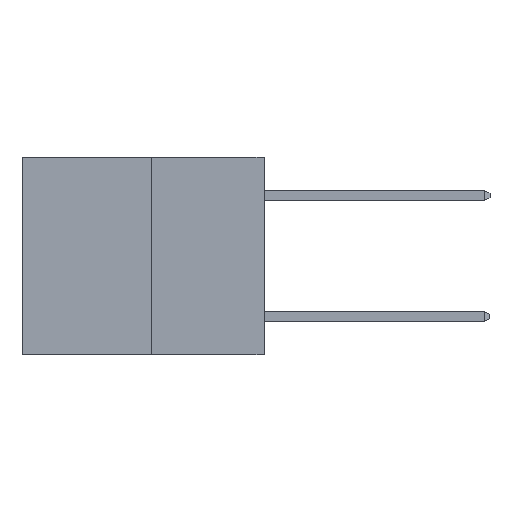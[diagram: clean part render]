
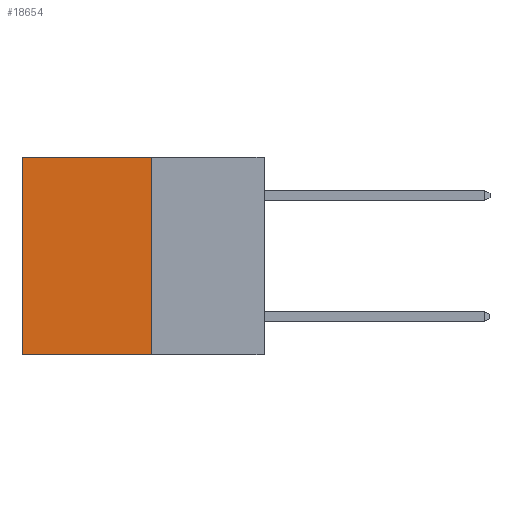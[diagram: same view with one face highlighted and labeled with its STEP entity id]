
A CAD part, left-side view. The second image highlights one B-rep face of the part: STEP entity #18654.
In plain terms, the highlighted planar face has unit normal (-1, 0, 0).
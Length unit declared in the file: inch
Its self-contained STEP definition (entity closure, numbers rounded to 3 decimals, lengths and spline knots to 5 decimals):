
#894 = CARTESIAN_POINT ( 'NONE',  ( 0.3165, 0.6, 0. ) ) ;
#2401 = DIRECTION ( 'NONE',  ( 0., 0., -1. ) ) ;
#2449 = VERTEX_POINT ( 'NONE', #3518 ) ;
#2598 = VECTOR ( 'NONE', #17071, 39.37008 ) ;
#3518 = CARTESIAN_POINT ( 'NONE',  ( 0.3165, 0.28, -0.49 ) ) ;
#3883 = LINE ( 'NONE', #11836, #6253 ) ;
#4028 = EDGE_LOOP ( 'NONE', ( #17519, #9952, #17706, #15901 ) ) ;
#4644 = CARTESIAN_POINT ( 'NONE',  ( 0.3165, 0.28, 0. ) ) ;
#5313 = CARTESIAN_POINT ( 'NONE',  ( 0.3165, 0.6, -0.49 ) ) ;
#6253 = VECTOR ( 'NONE', #16473, 39.37008 ) ;
#6713 = DIRECTION ( 'NONE',  ( 0., 0., -1. ) ) ;
#6855 = EDGE_CURVE ( 'NONE', #7394, #12419, #11944, .T. ) ;
#7394 = VERTEX_POINT ( 'NONE', #17619 ) ;
#7430 = LINE ( 'NONE', #15660, #16113 ) ;
#8497 = PLANE ( 'NONE',  #19822 ) ;
#9324 = EDGE_CURVE ( 'NONE', #7394, #2449, #10800, .T. ) ;
#9455 = FACE_OUTER_BOUND ( 'NONE', #4028, .T. ) ;
#9952 = ORIENTED_EDGE ( 'NONE', *, *, #15131, .F. ) ;
#10045 = CARTESIAN_POINT ( 'NONE',  ( 0.3165, 0.28, -0.49 ) ) ;
#10800 = LINE ( 'NONE', #16528, #17772 ) ;
#11588 = DIRECTION ( 'NONE',  ( 1., 0., 0. ) ) ;
#11836 = CARTESIAN_POINT ( 'NONE',  ( 0.3165, 0.28, -0.49 ) ) ;
#11944 = LINE ( 'NONE', #4644, #2598 ) ;
#12419 = VERTEX_POINT ( 'NONE', #894 ) ;
#15131 = EDGE_CURVE ( 'NONE', #2449, #15538, #3883, .T. ) ;
#15538 = VERTEX_POINT ( 'NONE', #5313 ) ;
#15660 = CARTESIAN_POINT ( 'NONE',  ( 0.3165, 0.6, -0.49 ) ) ;
#15847 = EDGE_CURVE ( 'NONE', #12419, #15538, #7430, .T. ) ;
#15901 = ORIENTED_EDGE ( 'NONE', *, *, #6855, .T. ) ;
#16113 = VECTOR ( 'NONE', #6713, 39.37008 ) ;
#16473 = DIRECTION ( 'NONE',  ( 0., 1., 0. ) ) ;
#16528 = CARTESIAN_POINT ( 'NONE',  ( 0.3165, 0.28, -0.49 ) ) ;
#16669 = DIRECTION ( 'NONE',  ( 0., 0., -1. ) ) ;
#17071 = DIRECTION ( 'NONE',  ( 0., 1., 0. ) ) ;
#17519 = ORIENTED_EDGE ( 'NONE', *, *, #15847, .T. ) ;
#17619 = CARTESIAN_POINT ( 'NONE',  ( 0.3165, 0.28, 0. ) ) ;
#17706 = ORIENTED_EDGE ( 'NONE', *, *, #9324, .F. ) ;
#17772 = VECTOR ( 'NONE', #16669, 39.37008 ) ;
#18654 = ADVANCED_FACE ( 'NONE', ( #9455 ), #8497, .F. ) ;
#19822 = AXIS2_PLACEMENT_3D ( 'NONE', #10045, #11588, #2401 ) ;
